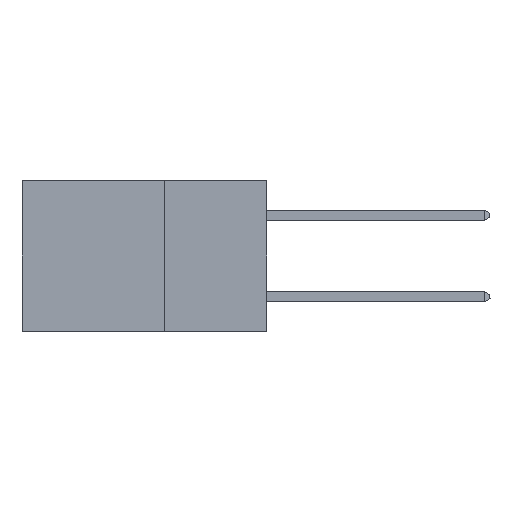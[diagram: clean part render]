
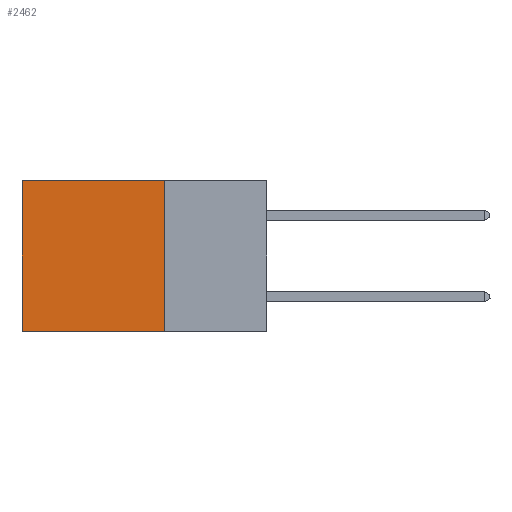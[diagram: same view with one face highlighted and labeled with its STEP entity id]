
A CAD part, left-side view. The second image highlights one B-rep face of the part: STEP entity #2462.
In plain terms, the highlighted planar face has unit normal (-1, 0, 0).
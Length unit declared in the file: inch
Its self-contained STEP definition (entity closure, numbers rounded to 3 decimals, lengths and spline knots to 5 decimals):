
#276 = VECTOR ( 'NONE', #4227, 39.37008 ) ;
#432 = VERTEX_POINT ( 'NONE', #5781 ) ;
#1940 = CARTESIAN_POINT ( 'NONE',  ( 0.2875, 0.25, 0. ) ) ;
#2462 = ADVANCED_FACE ( 'NONE', ( #35240 ), #21753, .F. ) ;
#4132 = EDGE_CURVE ( 'NONE', #18509, #11470, #15710, .T. ) ;
#4227 = DIRECTION ( 'NONE',  ( 0., 0., -1. ) ) ;
#5781 = CARTESIAN_POINT ( 'NONE',  ( 0.2875, 0.6, -0.37 ) ) ;
#6857 = ORIENTED_EDGE ( 'NONE', *, *, #28469, .T. ) ;
#8449 = VECTOR ( 'NONE', #27404, 39.37008 ) ;
#8497 = EDGE_CURVE ( 'NONE', #18509, #34751, #26668, .T. ) ;
#10243 = VECTOR ( 'NONE', #14992, 39.37008 ) ;
#11470 = VERTEX_POINT ( 'NONE', #14628 ) ;
#12793 = LINE ( 'NONE', #28903, #10243 ) ;
#13639 = DIRECTION ( 'NONE',  ( 1., 0., 0. ) ) ;
#14628 = CARTESIAN_POINT ( 'NONE',  ( 0.2875, 0.6, 0. ) ) ;
#14992 = DIRECTION ( 'NONE',  ( 0., 1., 0. ) ) ;
#15202 = EDGE_LOOP ( 'NONE', ( #6857, #19616, #18527, #25807 ) ) ;
#15209 = CARTESIAN_POINT ( 'NONE',  ( 0.2875, 0.6, 0. ) ) ;
#15710 = LINE ( 'NONE', #1940, #8449 ) ;
#18169 = AXIS2_PLACEMENT_3D ( 'NONE', #35569, #13639, #18846 ) ;
#18509 = VERTEX_POINT ( 'NONE', #31511 ) ;
#18527 = ORIENTED_EDGE ( 'NONE', *, *, #8497, .F. ) ;
#18846 = DIRECTION ( 'NONE',  ( 0., 0., -1. ) ) ;
#19616 = ORIENTED_EDGE ( 'NONE', *, *, #33479, .F. ) ;
#21753 = PLANE ( 'NONE',  #18169 ) ;
#22770 = CARTESIAN_POINT ( 'NONE',  ( 0.2875, 0.25, -0.37 ) ) ;
#25318 = CARTESIAN_POINT ( 'NONE',  ( 0.2875, 0.25, 0. ) ) ;
#25807 = ORIENTED_EDGE ( 'NONE', *, *, #4132, .T. ) ;
#26668 = LINE ( 'NONE', #25318, #29712 ) ;
#27404 = DIRECTION ( 'NONE',  ( 0., 1., 0. ) ) ;
#28375 = DIRECTION ( 'NONE',  ( 0., 0., -1. ) ) ;
#28469 = EDGE_CURVE ( 'NONE', #11470, #432, #34698, .T. ) ;
#28903 = CARTESIAN_POINT ( 'NONE',  ( 0.2875, 0.25, -0.37 ) ) ;
#29712 = VECTOR ( 'NONE', #28375, 39.37008 ) ;
#31511 = CARTESIAN_POINT ( 'NONE',  ( 0.2875, 0.25, 0. ) ) ;
#33479 = EDGE_CURVE ( 'NONE', #34751, #432, #12793, .T. ) ;
#34698 = LINE ( 'NONE', #15209, #276 ) ;
#34751 = VERTEX_POINT ( 'NONE', #22770 ) ;
#35240 = FACE_OUTER_BOUND ( 'NONE', #15202, .T. ) ;
#35569 = CARTESIAN_POINT ( 'NONE',  ( 0.2875, 0.25, 0. ) ) ;
